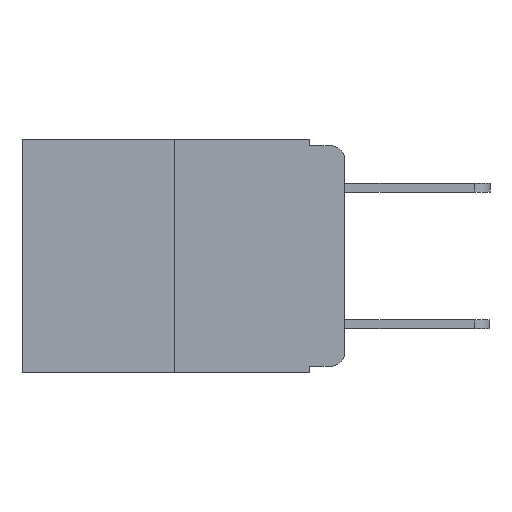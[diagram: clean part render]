
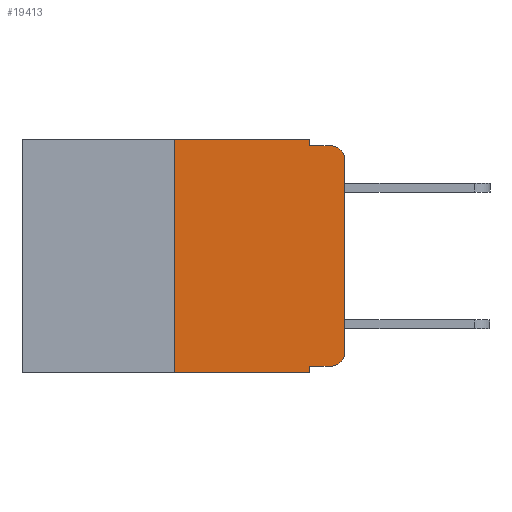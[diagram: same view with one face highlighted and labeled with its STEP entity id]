
A CAD part, left-side view. The second image highlights one B-rep face of the part: STEP entity #19413.
In plain terms, the highlighted planar face has unit normal (-1, 0, 0).
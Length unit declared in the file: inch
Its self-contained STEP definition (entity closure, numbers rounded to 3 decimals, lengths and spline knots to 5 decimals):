
#414 = DIRECTION ( 'NONE',  ( 0., 0., -1. ) ) ;
#654 = VECTOR ( 'NONE', #23399, 39.37008 ) ;
#737 = EDGE_LOOP ( 'NONE', ( #15165, #12640, #15233, #12005, #919, #2308, #3327, #1311, #2870, #8158 ) ) ;
#919 = ORIENTED_EDGE ( 'NONE', *, *, #1663, .F. ) ;
#1311 = ORIENTED_EDGE ( 'NONE', *, *, #19650, .F. ) ;
#1570 = EDGE_CURVE ( 'NONE', #24031, #14854, #13476, .T. ) ;
#1661 = CARTESIAN_POINT ( 'NONE',  ( 0., 0.473, -0.343 ) ) ;
#1663 = EDGE_CURVE ( 'NONE', #7940, #3863, #11780, .T. ) ;
#2305 = CARTESIAN_POINT ( 'NONE',  ( 0., 0., -0.03 ) ) ;
#2308 = ORIENTED_EDGE ( 'NONE', *, *, #12565, .F. ) ;
#2566 = CARTESIAN_POINT ( 'NONE',  ( 0., 0.051, 0. ) ) ;
#2859 = CARTESIAN_POINT ( 'NONE',  ( 0., 0.25, -0.343 ) ) ;
#2870 = ORIENTED_EDGE ( 'NONE', *, *, #16967, .T. ) ;
#3327 = ORIENTED_EDGE ( 'NONE', *, *, #5605, .T. ) ;
#3352 = VECTOR ( 'NONE', #414, 39.37008 ) ;
#3863 = VERTEX_POINT ( 'NONE', #2566 ) ;
#4382 = VERTEX_POINT ( 'NONE', #22248 ) ;
#5116 = LINE ( 'NONE', #7209, #23572 ) ;
#5407 = DIRECTION ( 'NONE',  ( 0., 0., 1. ) ) ;
#5605 = EDGE_CURVE ( 'NONE', #19171, #23988, #16225, .T. ) ;
#5640 = DIRECTION ( 'NONE',  ( 0., 0., -1. ) ) ;
#5768 = DIRECTION ( 'NONE',  ( 0., 0., 1. ) ) ;
#5943 = VECTOR ( 'NONE', #7652, 39.37008 ) ;
#7061 = EDGE_CURVE ( 'NONE', #3863, #15523, #14460, .T. ) ;
#7209 = CARTESIAN_POINT ( 'NONE',  ( 0., 0.051, -0.01 ) ) ;
#7652 = DIRECTION ( 'NONE',  ( 0., -1., 0. ) ) ;
#7749 = CARTESIAN_POINT ( 'NONE',  ( 0., 0., 0. ) ) ;
#7940 = VERTEX_POINT ( 'NONE', #15486 ) ;
#8003 = LINE ( 'NONE', #11944, #3352 ) ;
#8158 = ORIENTED_EDGE ( 'NONE', *, *, #11808, .T. ) ;
#8980 = EDGE_CURVE ( 'NONE', #19071, #24031, #16635, .T. ) ;
#9101 = DIRECTION ( 'NONE',  ( 0., -1., 0. ) ) ;
#9443 = EDGE_CURVE ( 'NONE', #15523, #14854, #5116, .T. ) ;
#9605 = VECTOR ( 'NONE', #5768, 39.37008 ) ;
#10609 = DIRECTION ( 'NONE',  ( -1., 0., 0. ) ) ;
#11329 = CARTESIAN_POINT ( 'NONE',  ( 0., 0.473, 0. ) ) ;
#11383 = DIRECTION ( 'NONE',  ( 0., -1., 0. ) ) ;
#11780 = LINE ( 'NONE', #11329, #15979 ) ;
#11808 = EDGE_CURVE ( 'NONE', #4382, #19071, #15058, .T. ) ;
#11944 = CARTESIAN_POINT ( 'NONE',  ( 0., 0.051, 0. ) ) ;
#12005 = ORIENTED_EDGE ( 'NONE', *, *, #7061, .F. ) ;
#12224 = AXIS2_PLACEMENT_3D ( 'NONE', #21564, #10609, #23407 ) ;
#12296 = AXIS2_PLACEMENT_3D ( 'NONE', #15503, #15455, #19044 ) ;
#12565 = EDGE_CURVE ( 'NONE', #19171, #7940, #16475, .T. ) ;
#12640 = ORIENTED_EDGE ( 'NONE', *, *, #1570, .T. ) ;
#12861 = CARTESIAN_POINT ( 'NONE',  ( 0., 0.051, -0.333 ) ) ;
#13476 = CIRCLE ( 'NONE', #12296, 0.02 ) ;
#13854 = CARTESIAN_POINT ( 'NONE',  ( 0., 0., -0.313 ) ) ;
#14460 = LINE ( 'NONE', #15461, #23701 ) ;
#14763 = CARTESIAN_POINT ( 'NONE',  ( 0., 0.473, 0. ) ) ;
#14854 = VERTEX_POINT ( 'NONE', #17635 ) ;
#15058 = CIRCLE ( 'NONE', #12224, 0.02 ) ;
#15165 = ORIENTED_EDGE ( 'NONE', *, *, #8980, .T. ) ;
#15233 = ORIENTED_EDGE ( 'NONE', *, *, #9443, .F. ) ;
#15455 = DIRECTION ( 'NONE',  ( -1., 0., 0. ) ) ;
#15461 = CARTESIAN_POINT ( 'NONE',  ( 0., 0.051, 0. ) ) ;
#15486 = CARTESIAN_POINT ( 'NONE',  ( 0., 0.25, 0. ) ) ;
#15503 = CARTESIAN_POINT ( 'NONE',  ( 0., 0.02, -0.03 ) ) ;
#15523 = VERTEX_POINT ( 'NONE', #21841 ) ;
#15979 = VECTOR ( 'NONE', #11383, 39.37008 ) ;
#16225 = LINE ( 'NONE', #1661, #5943 ) ;
#16304 = CARTESIAN_POINT ( 'NONE',  ( 0., 0.25, 0. ) ) ;
#16475 = LINE ( 'NONE', #16304, #20876 ) ;
#16609 = DIRECTION ( 'NONE',  ( 1., 0., 0. ) ) ;
#16635 = LINE ( 'NONE', #7749, #9605 ) ;
#16967 = EDGE_CURVE ( 'NONE', #21502, #4382, #20098, .T. ) ;
#17055 = AXIS2_PLACEMENT_3D ( 'NONE', #14763, #16609, #5640 ) ;
#17327 = DIRECTION ( 'NONE',  ( 0., 0., -1. ) ) ;
#17635 = CARTESIAN_POINT ( 'NONE',  ( 0., 0.02, -0.01 ) ) ;
#18972 = CARTESIAN_POINT ( 'NONE',  ( 0., 0.051, -0.343 ) ) ;
#19044 = DIRECTION ( 'NONE',  ( 0., 0., -1. ) ) ;
#19071 = VERTEX_POINT ( 'NONE', #13854 ) ;
#19103 = FACE_OUTER_BOUND ( 'NONE', #737, .T. ) ;
#19171 = VERTEX_POINT ( 'NONE', #2859 ) ;
#19413 = ADVANCED_FACE ( 'NONE', ( #19103 ), #23970, .F. ) ;
#19650 = EDGE_CURVE ( 'NONE', #21502, #23988, #8003, .T. ) ;
#20098 = LINE ( 'NONE', #21559, #654 ) ;
#20876 = VECTOR ( 'NONE', #5407, 39.37008 ) ;
#21502 = VERTEX_POINT ( 'NONE', #12861 ) ;
#21559 = CARTESIAN_POINT ( 'NONE',  ( 0., 0.051, -0.333 ) ) ;
#21564 = CARTESIAN_POINT ( 'NONE',  ( 0., 0.02, -0.313 ) ) ;
#21841 = CARTESIAN_POINT ( 'NONE',  ( 0., 0.051, -0.01 ) ) ;
#22248 = CARTESIAN_POINT ( 'NONE',  ( 0., 0.02, -0.333 ) ) ;
#23399 = DIRECTION ( 'NONE',  ( 0., -1., 0. ) ) ;
#23407 = DIRECTION ( 'NONE',  ( 0., 0., -1. ) ) ;
#23572 = VECTOR ( 'NONE', #9101, 39.37008 ) ;
#23701 = VECTOR ( 'NONE', #17327, 39.37008 ) ;
#23970 = PLANE ( 'NONE',  #17055 ) ;
#23988 = VERTEX_POINT ( 'NONE', #18972 ) ;
#24031 = VERTEX_POINT ( 'NONE', #2305 ) ;
